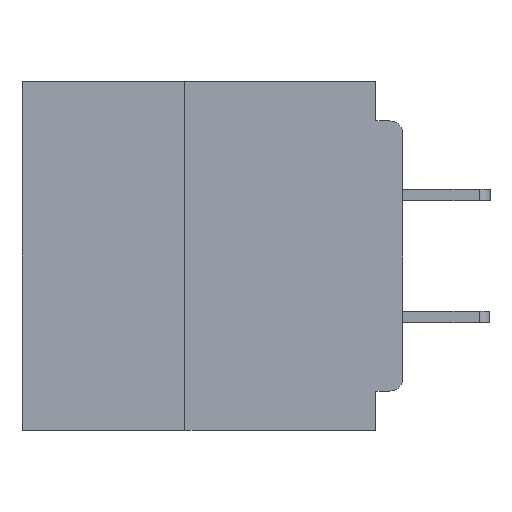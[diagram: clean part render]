
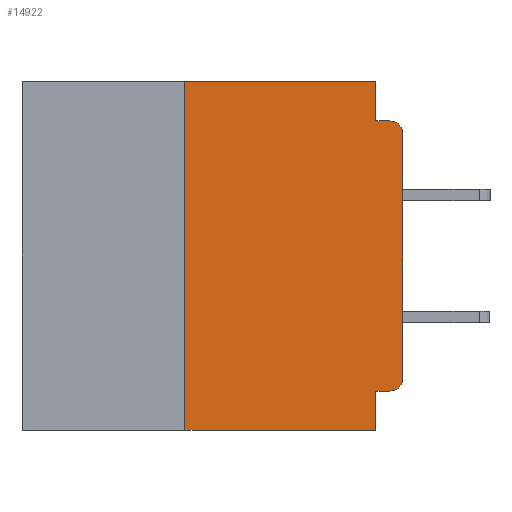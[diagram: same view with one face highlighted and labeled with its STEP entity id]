
A CAD part, left-side view. The second image highlights one B-rep face of the part: STEP entity #14922.
In plain terms, the highlighted planar face has unit normal (-1, 0, 0).
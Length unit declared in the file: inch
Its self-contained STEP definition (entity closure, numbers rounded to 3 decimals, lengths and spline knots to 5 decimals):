
#445 = EDGE_CURVE ( 'NONE', #27794, #27178, #34723, .T. ) ;
#985 = VERTEX_POINT ( 'NONE', #25816 ) ;
#1416 = FACE_OUTER_BOUND ( 'NONE', #19550, .T. ) ;
#1636 = CARTESIAN_POINT ( 'NONE',  ( 0., 0.25, -0.4 ) ) ;
#1951 = CARTESIAN_POINT ( 'NONE',  ( 0., 0.031, 0. ) ) ;
#2300 = ORIENTED_EDGE ( 'NONE', *, *, #33601, .F. ) ;
#3193 = ORIENTED_EDGE ( 'NONE', *, *, #22147, .T. ) ;
#3632 = CARTESIAN_POINT ( 'NONE',  ( 0., 0., -0.045 ) ) ;
#4256 = DIRECTION ( 'NONE',  ( 0., 0., -1. ) ) ;
#4564 = CARTESIAN_POINT ( 'NONE',  ( 0., 0.437, 0. ) ) ;
#4914 = ORIENTED_EDGE ( 'NONE', *, *, #41306, .F. ) ;
#5305 = DIRECTION ( 'NONE',  ( 0., -1., 0. ) ) ;
#7410 = ORIENTED_EDGE ( 'NONE', *, *, #37495, .T. ) ;
#7501 = CARTESIAN_POINT ( 'NONE',  ( 0., 0.015, -0.045 ) ) ;
#8515 = CIRCLE ( 'NONE', #9839, 0.015 ) ;
#8669 = LINE ( 'NONE', #3632, #42295 ) ;
#9140 = LINE ( 'NONE', #38731, #25466 ) ;
#9839 = AXIS2_PLACEMENT_3D ( 'NONE', #38068, #18547, #41348 ) ;
#11226 = DIRECTION ( 'NONE',  ( 0., 0., -1. ) ) ;
#11766 = ORIENTED_EDGE ( 'NONE', *, *, #25748, .T. ) ;
#11928 = CARTESIAN_POINT ( 'NONE',  ( 0., 0.25, 0. ) ) ;
#13682 = ORIENTED_EDGE ( 'NONE', *, *, #37107, .T. ) ;
#13896 = DIRECTION ( 'NONE',  ( 0., 0., 1. ) ) ;
#14757 = DIRECTION ( 'NONE',  ( -1., 0., 0. ) ) ;
#14922 = ADVANCED_FACE ( 'NONE', ( #1416 ), #20863, .F. ) ;
#15245 = VERTEX_POINT ( 'NONE', #22544 ) ;
#16610 = CARTESIAN_POINT ( 'NONE',  ( 0., 0.031, -0.355 ) ) ;
#16823 = VECTOR ( 'NONE', #4256, 39.37008 ) ;
#16996 = CARTESIAN_POINT ( 'NONE',  ( 0., 0.015, -0.355 ) ) ;
#17294 = CARTESIAN_POINT ( 'NONE',  ( 0., 0.031, -0.4 ) ) ;
#17377 = VECTOR ( 'NONE', #37390, 39.37008 ) ;
#18414 = LINE ( 'NONE', #22748, #27132 ) ;
#18547 = DIRECTION ( 'NONE',  ( -1., 0., 0. ) ) ;
#19328 = DIRECTION ( 'NONE',  ( 0., -1., 0. ) ) ;
#19550 = EDGE_LOOP ( 'NONE', ( #7410, #11766, #4914, #29762, #39003, #40011, #13682, #2300, #40167, #3193 ) ) ;
#20211 = VERTEX_POINT ( 'NONE', #41216 ) ;
#20863 = PLANE ( 'NONE',  #34683 ) ;
#21004 = EDGE_CURVE ( 'NONE', #22067, #24006, #9140, .T. ) ;
#21068 = EDGE_CURVE ( 'NONE', #30707, #31910, #40732, .T. ) ;
#21278 = LINE ( 'NONE', #37833, #28991 ) ;
#22067 = VERTEX_POINT ( 'NONE', #1636 ) ;
#22147 = EDGE_CURVE ( 'NONE', #30707, #20211, #8515, .T. ) ;
#22265 = VECTOR ( 'NONE', #13896, 39.37008 ) ;
#22485 = DIRECTION ( 'NONE',  ( 0., 0., 1. ) ) ;
#22544 = CARTESIAN_POINT ( 'NONE',  ( 0., 0., -0.06 ) ) ;
#22748 = CARTESIAN_POINT ( 'NONE',  ( 0., 0.437, 0. ) ) ;
#22759 = CARTESIAN_POINT ( 'NONE',  ( 0., 0., -0.355 ) ) ;
#24006 = VERTEX_POINT ( 'NONE', #11928 ) ;
#25466 = VECTOR ( 'NONE', #22485, 39.37008 ) ;
#25525 = LINE ( 'NONE', #17294, #16823 ) ;
#25748 = EDGE_CURVE ( 'NONE', #15245, #36908, #34033, .T. ) ;
#25816 = CARTESIAN_POINT ( 'NONE',  ( 0., 0.031, -0.4 ) ) ;
#27132 = VECTOR ( 'NONE', #19328, 39.37008 ) ;
#27178 = VERTEX_POINT ( 'NONE', #39589 ) ;
#27794 = VERTEX_POINT ( 'NONE', #36106 ) ;
#28991 = VECTOR ( 'NONE', #5305, 39.37008 ) ;
#29762 = ORIENTED_EDGE ( 'NONE', *, *, #445, .F. ) ;
#30006 = CARTESIAN_POINT ( 'NONE',  ( 0., 0., 0. ) ) ;
#30707 = VERTEX_POINT ( 'NONE', #16996 ) ;
#30745 = DIRECTION ( 'NONE',  ( 1., 0., 0. ) ) ;
#31008 = LINE ( 'NONE', #30006, #22265 ) ;
#31910 = VERTEX_POINT ( 'NONE', #16610 ) ;
#32894 = AXIS2_PLACEMENT_3D ( 'NONE', #34280, #14757, #37521 ) ;
#32896 = EDGE_CURVE ( 'NONE', #24006, #27794, #18414, .T. ) ;
#33601 = EDGE_CURVE ( 'NONE', #31910, #985, #25525, .T. ) ;
#34033 = CIRCLE ( 'NONE', #32894, 0.015 ) ;
#34280 = CARTESIAN_POINT ( 'NONE',  ( 0., 0.015, -0.06 ) ) ;
#34683 = AXIS2_PLACEMENT_3D ( 'NONE', #4564, #30745, #11226 ) ;
#34723 = LINE ( 'NONE', #1951, #17377 ) ;
#35869 = DIRECTION ( 'NONE',  ( 0., 1., 0. ) ) ;
#36106 = CARTESIAN_POINT ( 'NONE',  ( 0., 0.031, 0. ) ) ;
#36908 = VERTEX_POINT ( 'NONE', #7501 ) ;
#37107 = EDGE_CURVE ( 'NONE', #22067, #985, #21278, .T. ) ;
#37390 = DIRECTION ( 'NONE',  ( 0., 0., -1. ) ) ;
#37495 = EDGE_CURVE ( 'NONE', #20211, #15245, #31008, .T. ) ;
#37521 = DIRECTION ( 'NONE',  ( 0., 0., -1. ) ) ;
#37833 = CARTESIAN_POINT ( 'NONE',  ( 0., 0.437, -0.4 ) ) ;
#38068 = CARTESIAN_POINT ( 'NONE',  ( 0., 0.015, -0.34 ) ) ;
#38675 = VECTOR ( 'NONE', #35869, 39.37008 ) ;
#38731 = CARTESIAN_POINT ( 'NONE',  ( 0., 0.25, -0.4 ) ) ;
#39003 = ORIENTED_EDGE ( 'NONE', *, *, #32896, .F. ) ;
#39589 = CARTESIAN_POINT ( 'NONE',  ( 0., 0.031, -0.045 ) ) ;
#39619 = DIRECTION ( 'NONE',  ( 0., -1., 0. ) ) ;
#40011 = ORIENTED_EDGE ( 'NONE', *, *, #21004, .F. ) ;
#40167 = ORIENTED_EDGE ( 'NONE', *, *, #21068, .F. ) ;
#40732 = LINE ( 'NONE', #22759, #38675 ) ;
#41216 = CARTESIAN_POINT ( 'NONE',  ( 0., 0., -0.34 ) ) ;
#41306 = EDGE_CURVE ( 'NONE', #27178, #36908, #8669, .T. ) ;
#41348 = DIRECTION ( 'NONE',  ( 0., 0., -1. ) ) ;
#42295 = VECTOR ( 'NONE', #39619, 39.37008 ) ;
